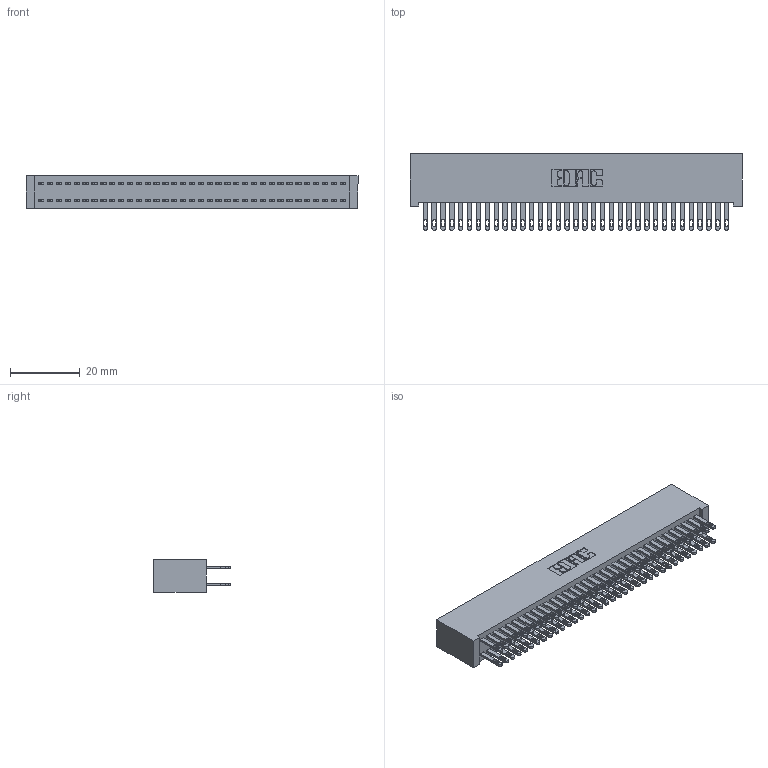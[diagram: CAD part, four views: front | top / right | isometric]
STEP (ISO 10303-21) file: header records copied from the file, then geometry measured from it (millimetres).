
FILE_DESCRIPTION (( 'STEP AP203' ), '1' );
FILE_NAME ('342-070-500-201.STEP', '2019-10-03T15:48:01', ( '' ), ( '' ), 'SwSTEP 2.0', 'SolidWorks 2016', '' );
FILE_SCHEMA (( 'CONFIG_CONTROL_DESIGN' ));
Length unit declared in the file: inch
Products named in the file (3): 342 Part_Lugless; 345-292-001_345-293-100; 342-070-500-201
Assembly tree (71 placements, depth 2):
  342-070-500-201
    342 Part_Lugless
    345-292-001_345-293-100  x70
Bounding box: 95.15 x 21.85 x 9.4 mm (x, y, z)
Volume: 9169.4 mm3; surface area: 15869.4 mm2
Topology: 71 solids, 71 shells, 3462 faces, 10565 edges, 7042 vertices
Faces by surface type: plane 2162, cylinder 1300
Entity records: 22943 total; most frequent: CARTESIAN_POINT 3806, ORIENTED_EDGE 3742, DIRECTION 3259, EDGE_CURVE 1871, VECTOR 1747, LINE 1747, VERTEX_POINT 1246, AXIS2_PLACEMENT_3D 756
